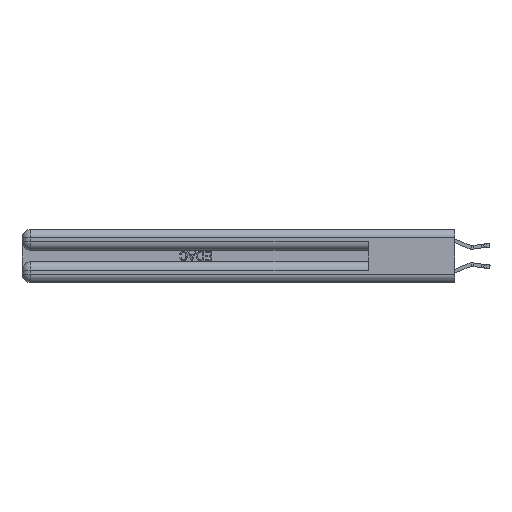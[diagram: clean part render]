
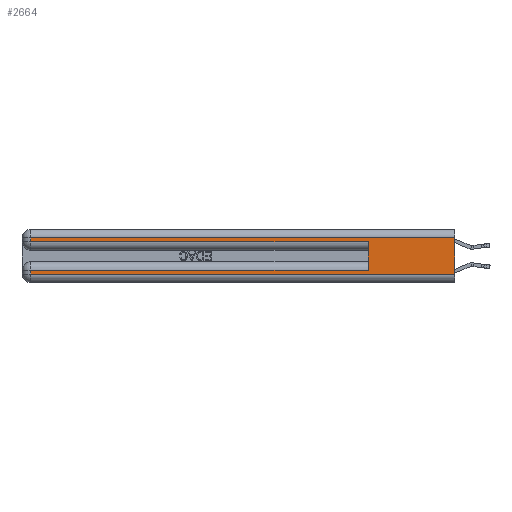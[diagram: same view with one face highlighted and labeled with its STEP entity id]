
A CAD part, left-side view. The second image highlights one B-rep face of the part: STEP entity #2664.
In plain terms, the highlighted planar face has unit normal (-1, 0, 0).
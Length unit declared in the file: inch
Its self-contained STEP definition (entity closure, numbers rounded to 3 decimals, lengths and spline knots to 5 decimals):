
#961 = EDGE_CURVE ( 'NONE', #27018, #18853, #24022, .T. ) ;
#1132 = VECTOR ( 'NONE', #23908, 39.37008 ) ;
#2664 = ADVANCED_FACE ( 'NONE', ( #7120 ), #26428, .F. ) ;
#2832 = AXIS2_PLACEMENT_3D ( 'NONE', #30151, #16253, #11444 ) ;
#3287 = DIRECTION ( 'NONE',  ( 0., 1., 0. ) ) ;
#7037 = ORIENTED_EDGE ( 'NONE', *, *, #26329, .T. ) ;
#7043 = ORIENTED_EDGE ( 'NONE', *, *, #27594, .T. ) ;
#7093 = CARTESIAN_POINT ( 'NONE',  ( 0., 0., 0.06 ) ) ;
#7120 = FACE_OUTER_BOUND ( 'NONE', #8744, .T. ) ;
#7691 = DIRECTION ( 'NONE',  ( 0., 1., 0. ) ) ;
#8510 = EDGE_CURVE ( 'NONE', #22594, #24613, #25922, .T. ) ;
#8692 = CARTESIAN_POINT ( 'NONE',  ( 0., 0., 0.06 ) ) ;
#8744 = EDGE_LOOP ( 'NONE', ( #10377, #7037, #24206, #32124, #19433, #7043, #10472, #30046 ) ) ;
#9027 = VECTOR ( 'NONE', #26870, 39.37008 ) ;
#9128 = VECTOR ( 'NONE', #11265, 39.37008 ) ;
#9242 = CARTESIAN_POINT ( 'NONE',  ( 0., 2.94, 0.37 ) ) ;
#9522 = CARTESIAN_POINT ( 'NONE',  ( 0., 2.94, 0.31 ) ) ;
#10377 = ORIENTED_EDGE ( 'NONE', *, *, #961, .F. ) ;
#10472 = ORIENTED_EDGE ( 'NONE', *, *, #23782, .T. ) ;
#11265 = DIRECTION ( 'NONE',  ( 0., 0., -1. ) ) ;
#11444 = DIRECTION ( 'NONE',  ( 0., 0., -1. ) ) ;
#12697 = LINE ( 'NONE', #9242, #19708 ) ;
#12783 = CARTESIAN_POINT ( 'NONE',  ( 0., 2.94, 0.285 ) ) ;
#13502 = CARTESIAN_POINT ( 'NONE',  ( 0., 0., 0.285 ) ) ;
#14102 = LINE ( 'NONE', #13502, #26584 ) ;
#14549 = VERTEX_POINT ( 'NONE', #23907 ) ;
#15167 = CARTESIAN_POINT ( 'NONE',  ( 0., 0.6, 0.285 ) ) ;
#15356 = CARTESIAN_POINT ( 'NONE',  ( 0., 0., 0.085 ) ) ;
#15493 = EDGE_CURVE ( 'NONE', #14549, #29129, #31313, .T. ) ;
#16253 = DIRECTION ( 'NONE',  ( 1., 0., 0. ) ) ;
#16282 = CARTESIAN_POINT ( 'NONE',  ( 0., 0.6, 0.145 ) ) ;
#17376 = VECTOR ( 'NONE', #17510, 39.37008 ) ;
#17510 = DIRECTION ( 'NONE',  ( 0., 0., -1. ) ) ;
#17624 = LINE ( 'NONE', #23089, #28583 ) ;
#18355 = CARTESIAN_POINT ( 'NONE',  ( 0., 0., 0.31 ) ) ;
#18360 = VECTOR ( 'NONE', #7691, 39.37008 ) ;
#18437 = EDGE_CURVE ( 'NONE', #23329, #18853, #31755, .T. ) ;
#18534 = DIRECTION ( 'NONE',  ( 0., 0., -1. ) ) ;
#18683 = CARTESIAN_POINT ( 'NONE',  ( 0., 2.94, 0.37 ) ) ;
#18853 = VERTEX_POINT ( 'NONE', #8692 ) ;
#19433 = ORIENTED_EDGE ( 'NONE', *, *, #15493, .F. ) ;
#19708 = VECTOR ( 'NONE', #18534, 39.37008 ) ;
#22594 = VERTEX_POINT ( 'NONE', #9522 ) ;
#23089 = CARTESIAN_POINT ( 'NONE',  ( 0., 0., 0.31 ) ) ;
#23329 = VERTEX_POINT ( 'NONE', #29714 ) ;
#23782 = EDGE_CURVE ( 'NONE', #32341, #23329, #12697, .T. ) ;
#23907 = CARTESIAN_POINT ( 'NONE',  ( 0., 0.6, 0.085 ) ) ;
#23908 = DIRECTION ( 'NONE',  ( 0., 0., 1. ) ) ;
#24022 = LINE ( 'NONE', #32403, #17376 ) ;
#24206 = ORIENTED_EDGE ( 'NONE', *, *, #8510, .T. ) ;
#24613 = VERTEX_POINT ( 'NONE', #12783 ) ;
#25922 = LINE ( 'NONE', #18683, #9128 ) ;
#26329 = EDGE_CURVE ( 'NONE', #27018, #22594, #17624, .T. ) ;
#26428 = PLANE ( 'NONE',  #2832 ) ;
#26584 = VECTOR ( 'NONE', #28463, 39.37008 ) ;
#26870 = DIRECTION ( 'NONE',  ( 0., -1., 0. ) ) ;
#27018 = VERTEX_POINT ( 'NONE', #18355 ) ;
#27594 = EDGE_CURVE ( 'NONE', #14549, #32341, #30092, .T. ) ;
#28463 = DIRECTION ( 'NONE',  ( 0., -1., 0. ) ) ;
#28583 = VECTOR ( 'NONE', #3287, 39.37008 ) ;
#29129 = VERTEX_POINT ( 'NONE', #15167 ) ;
#29714 = CARTESIAN_POINT ( 'NONE',  ( 0., 2.94, 0.06 ) ) ;
#29970 = EDGE_CURVE ( 'NONE', #24613, #29129, #14102, .T. ) ;
#30046 = ORIENTED_EDGE ( 'NONE', *, *, #18437, .T. ) ;
#30092 = LINE ( 'NONE', #15356, #18360 ) ;
#30151 = CARTESIAN_POINT ( 'NONE',  ( 0., 0., 0.37 ) ) ;
#31313 = LINE ( 'NONE', #16282, #1132 ) ;
#31755 = LINE ( 'NONE', #7093, #9027 ) ;
#32124 = ORIENTED_EDGE ( 'NONE', *, *, #29970, .T. ) ;
#32341 = VERTEX_POINT ( 'NONE', #32361 ) ;
#32361 = CARTESIAN_POINT ( 'NONE',  ( 0., 2.94, 0.085 ) ) ;
#32403 = CARTESIAN_POINT ( 'NONE',  ( 0., 0., 0.37 ) ) ;
